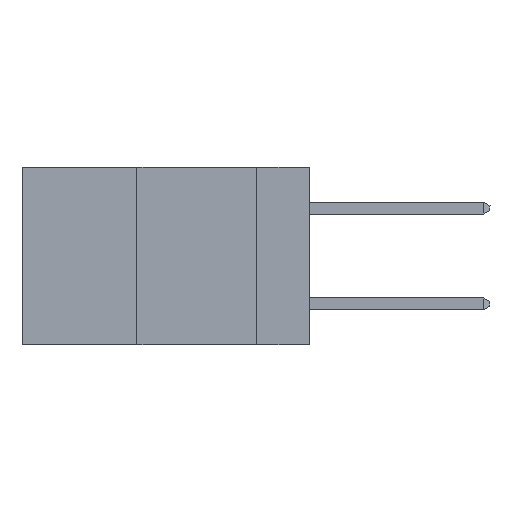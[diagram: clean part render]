
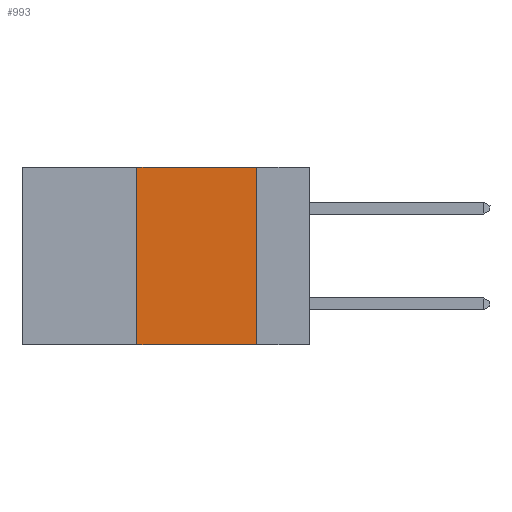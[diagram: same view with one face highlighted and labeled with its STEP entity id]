
A CAD part, left-side view. The second image highlights one B-rep face of the part: STEP entity #993.
In plain terms, the highlighted planar face has unit normal (-1, 0, 0).
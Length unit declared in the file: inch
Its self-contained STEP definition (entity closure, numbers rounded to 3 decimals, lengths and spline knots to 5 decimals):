
#225 = DIRECTION ( 'NONE',  ( 0., -1., 0. ) ) ;
#993 = ADVANCED_FACE ( 'NONE', ( #1176 ), #3343, .F. ) ;
#1098 = EDGE_LOOP ( 'NONE', ( #10811, #6237, #8822, #2428 ) ) ;
#1176 = FACE_OUTER_BOUND ( 'NONE', #1098, .T. ) ;
#1240 = DIRECTION ( 'NONE',  ( 0., 0., -1. ) ) ;
#1288 = DIRECTION ( 'NONE',  ( 1., 0., 0. ) ) ;
#2428 = ORIENTED_EDGE ( 'NONE', *, *, #6045, .T. ) ;
#2949 = LINE ( 'NONE', #13257, #11065 ) ;
#3343 = PLANE ( 'NONE',  #13658 ) ;
#3392 = VERTEX_POINT ( 'NONE', #8716 ) ;
#3661 = VERTEX_POINT ( 'NONE', #3816 ) ;
#3816 = CARTESIAN_POINT ( 'NONE',  ( 0., 0.11, 0. ) ) ;
#3838 = LINE ( 'NONE', #7187, #6456 ) ;
#4108 = CARTESIAN_POINT ( 'NONE',  ( 0., 0.36, 0. ) ) ;
#4336 = CARTESIAN_POINT ( 'NONE',  ( 0., 0.11, 0. ) ) ;
#4484 = DIRECTION ( 'NONE',  ( 0., -1., 0. ) ) ;
#5956 = EDGE_CURVE ( 'NONE', #3661, #3392, #12407, .T. ) ;
#6045 = EDGE_CURVE ( 'NONE', #7147, #3392, #2949, .T. ) ;
#6237 = ORIENTED_EDGE ( 'NONE', *, *, #7793, .F. ) ;
#6456 = VECTOR ( 'NONE', #12622, 39.37008 ) ;
#6814 = CARTESIAN_POINT ( 'NONE',  ( 0., 0.6, 0. ) ) ;
#7147 = VERTEX_POINT ( 'NONE', #9036 ) ;
#7187 = CARTESIAN_POINT ( 'NONE',  ( 0., 0.36, 0. ) ) ;
#7587 = LINE ( 'NONE', #6814, #13040 ) ;
#7793 = EDGE_CURVE ( 'NONE', #11282, #3661, #7587, .T. ) ;
#8716 = CARTESIAN_POINT ( 'NONE',  ( 0., 0.11, -0.37 ) ) ;
#8822 = ORIENTED_EDGE ( 'NONE', *, *, #12042, .F. ) ;
#9036 = CARTESIAN_POINT ( 'NONE',  ( 0., 0.36, -0.37 ) ) ;
#9504 = VECTOR ( 'NONE', #10968, 39.37008 ) ;
#10811 = ORIENTED_EDGE ( 'NONE', *, *, #5956, .F. ) ;
#10968 = DIRECTION ( 'NONE',  ( 0., 0., -1. ) ) ;
#11065 = VECTOR ( 'NONE', #4484, 39.37008 ) ;
#11282 = VERTEX_POINT ( 'NONE', #4108 ) ;
#12042 = EDGE_CURVE ( 'NONE', #7147, #11282, #3838, .T. ) ;
#12407 = LINE ( 'NONE', #4336, #9504 ) ;
#12622 = DIRECTION ( 'NONE',  ( 0., 0., 1. ) ) ;
#13040 = VECTOR ( 'NONE', #225, 39.37008 ) ;
#13127 = CARTESIAN_POINT ( 'NONE',  ( 0., 0.6, 0. ) ) ;
#13257 = CARTESIAN_POINT ( 'NONE',  ( 0., 0.6, -0.37 ) ) ;
#13658 = AXIS2_PLACEMENT_3D ( 'NONE', #13127, #1288, #1240 ) ;
